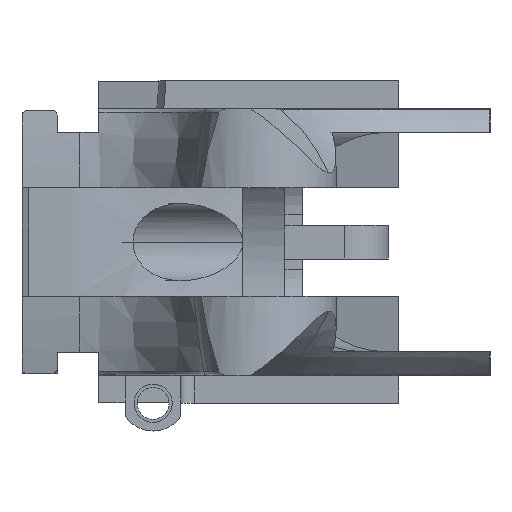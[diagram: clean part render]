
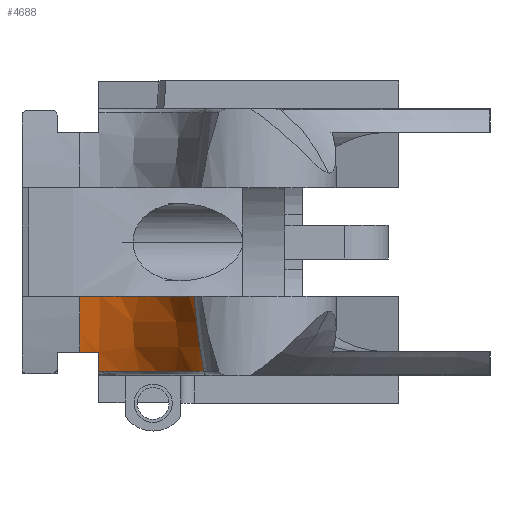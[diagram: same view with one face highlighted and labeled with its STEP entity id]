
A CAD part, left-side view. The second image highlights one B-rep face of the part: STEP entity #4688.
In plain terms, the highlighted free-form (B-spline) face has degree [3, 3] with [4, 4] control points.
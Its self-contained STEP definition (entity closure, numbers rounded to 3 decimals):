
#46 = CARTESIAN_POINT ( 'NONE',  ( -88.521, -1.184, -5.759 ) ) ;
#172 = EDGE_CURVE ( 'NONE', #8084, #7736, #11027, .T. ) ;
#174 = CARTESIAN_POINT ( 'NONE',  ( -77.615, -50.503, 0. ) ) ;
#343 = CARTESIAN_POINT ( 'NONE',  ( -80.423, 5.867, -9.367 ) ) ;
#382 = CARTESIAN_POINT ( 'NONE',  ( -85.981, -1.056, -9.367 ) ) ;
#948 = CARTESIAN_POINT ( 'NONE',  ( -80.848, 2.659, -7.57 ) ) ;
#1007 = CIRCLE ( 'NONE', #6863, 9.392 ) ;
#1082 = DIRECTION ( 'NONE',  ( 0., 0., 1. ) ) ;
#1248 = CARTESIAN_POINT ( 'NONE',  ( -30.319, 7.237, 0. ) ) ;
#1277 = CARTESIAN_POINT ( 'NONE',  ( -87.367, -1.543, -9.367 ) ) ;
#1711 = CARTESIAN_POINT ( 'NONE',  ( -88.325, -1.736, -9.367 ) ) ;
#1758 = CARTESIAN_POINT ( 'NONE',  ( -88.325, -1.736, -9.367 ) ) ;
#1840 = CARTESIAN_POINT ( 'NONE',  ( -88.472, -1.419, -7.57 ) ) ;
#1937 = EDGE_CURVE ( 'NONE', #3901, #10602, #9579, .T. ) ;
#1997 = EDGE_CURVE ( 'NONE', #3901, #7877, #7522, .T. ) ;
#2120 = ORIENTED_EDGE ( 'NONE', *, *, #172, .T. ) ;
#2134 = CARTESIAN_POINT ( 'NONE',  ( -80.652, 4.92, -9.367 ) ) ;
#2142 = DIRECTION ( 'NONE',  ( 0., 0., 1. ) ) ;
#2167 = CARTESIAN_POINT ( 'NONE',  ( -88.325, -1.736, -9.367 ) ) ;
#2214 = AXIS2_PLACEMENT_3D ( 'NONE', #7499, #2228, #8372 ) ;
#2228 = DIRECTION ( 'NONE',  ( 0., 0., 1. ) ) ;
#2232 = CARTESIAN_POINT ( 'NONE',  ( -88.325, -1.736, -9.367 ) ) ;
#2313 = EDGE_CURVE ( 'NONE', #7877, #11165, #3927, .T. ) ;
#2441 = EDGE_CURVE ( 'NONE', #8084, #11165, #6672, .T. ) ;
#2540 = EDGE_CURVE ( 'NONE', #7736, #2739, #8155, .T. ) ;
#2553 = ORIENTED_EDGE ( 'NONE', *, *, #1937, .F. ) ;
#2558 = CARTESIAN_POINT ( 'NONE',  ( -88.479, -1.035, -3.937 ) ) ;
#2729 = CARTESIAN_POINT ( 'NONE',  ( -80.511, 2.493, -9.367 ) ) ;
#2739 = VERTEX_POINT ( 'NONE', #9456 ) ;
#2751 = EDGE_CURVE ( 'NONE', #10602, #2739, #1007, .T. ) ;
#3018 = CARTESIAN_POINT ( 'NONE',  ( -80.994, 4.011, -9.367 ) ) ;
#3075 = CARTESIAN_POINT ( 'NONE',  ( -80.423, 5.867, -9.367 ) ) ;
#3589 = CARTESIAN_POINT ( 'NONE',  ( -84.2, -0.397, -3.937 ) ) ;
#3627 = CARTESIAN_POINT ( 'NONE',  ( -88.402, -1.748, -9.367 ) ) ;
#3901 = VERTEX_POINT ( 'NONE', #5484 ) ;
#3913 = CARTESIAN_POINT ( 'NONE',  ( -81.305, 3.348, -9.367 ) ) ;
#3927 = B_SPLINE_CURVE_WITH_KNOTS ( 'NONE', 3,
 ( #1711, #5273, #7034, #1758 ),
 .UNSPECIFIED., .F., .F.,
 ( 4, 4 ),
 ( 0., 0. ),
 .UNSPECIFIED. ) ;
#4460 = CARTESIAN_POINT ( 'NONE',  ( -80.824, 7.237, -5.759 ) ) ;
#4688 = ADVANCED_FACE ( 'NONE', ( #5041 ), #5638, .T. ) ;
#4791 = CARTESIAN_POINT ( 'NONE',  ( -82.477, 1.514, -9.367 ) ) ;
#4824 = EDGE_LOOP ( 'NONE', ( #2553, #7483, #10392, #8589, #2120, #7102, #5595 ) ) ;
#4846 = CARTESIAN_POINT ( 'NONE',  ( -80.669, 5.867, -7.976 ) ) ;
#5041 = FACE_OUTER_BOUND ( 'NONE', #4824, .T. ) ;
#5125 = CARTESIAN_POINT ( 'NONE',  ( -89.865, 7.772, -7.976 ) ) ;
#5273 = CARTESIAN_POINT ( 'NONE',  ( -88.325, -1.736, -9.367 ) ) ;
#5318 = AXIS2_PLACEMENT_3D ( 'NONE', #174, #6374, #1082 ) ;
#5368 = CARTESIAN_POINT ( 'NONE',  ( -84.102, -0.521, -5.759 ) ) ;
#5484 = CARTESIAN_POINT ( 'NONE',  ( -80.423, 5.867, -9.367 ) ) ;
#5595 = ORIENTED_EDGE ( 'NONE', *, *, #2751, .F. ) ;
#5638 =( BOUNDED_SURFACE ( )  B_SPLINE_SURFACE ( 3, 3, ( 
 ( #7963, #9682, #3589, #9730 ),
 ( #4460, #10614, #5368, #46 ),
 ( #6250, #948, #7124, #1840 ),
 ( #7998, #2729, #8875, #3627 ) ),
 .UNSPECIFIED., .F., .F., .F. ) 
 B_SPLINE_SURFACE_WITH_KNOTS ( ( 4, 4 ),
 ( 4, 4 ),
 ( 0., 1. ),
 ( 0., 1. ),
 .UNSPECIFIED. ) 
 GEOMETRIC_REPRESENTATION_ITEM ( )  RATIONAL_B_SPLINE_SURFACE ( (
 ( 1., 0.851, 0.851, 1.),
 ( 0.999, 0.85, 0.85, 0.999),
 ( 0.999, 0.85, 0.85, 0.999),
 ( 1., 0.851, 0.851, 1.) ) ) 
 REPRESENTATION_ITEM ( '' )  SURFACE ( )  );
#5662 = CARTESIAN_POINT ( 'NONE',  ( -80.52, 5.388, -9.367 ) ) ;
#5700 = CARTESIAN_POINT ( 'NONE',  ( -84.676, -0.401, -9.367 ) ) ;
#6013 = DIRECTION ( 'NONE',  ( -1., 0., 0. ) ) ;
#6250 = CARTESIAN_POINT ( 'NONE',  ( -80.585, 7.237, -7.57 ) ) ;
#6374 = DIRECTION ( 'NONE',  ( -0.977, -0.214, 0. ) ) ;
#6573 = CARTESIAN_POINT ( 'NONE',  ( -86.437, -1.243, -9.367 ) ) ;
#6672 = CIRCLE ( 'NONE', #5318, 50.8 ) ;
#6859 = CARTESIAN_POINT ( 'NONE',  ( -80.669, 5.867, -7.976 ) ) ;
#6863 = AXIS2_PLACEMENT_3D ( 'NONE', #5125, #11261, #6013 ) ;
#7034 = CARTESIAN_POINT ( 'NONE',  ( -88.325, -1.736, -9.367 ) ) ;
#7102 = ORIENTED_EDGE ( 'NONE', *, *, #2540, .T. ) ;
#7124 = CARTESIAN_POINT ( 'NONE',  ( -83.937, -0.731, -7.57 ) ) ;
#7404 = DIRECTION ( 'NONE',  ( 0., -1., 0. ) ) ;
#7434 = CARTESIAN_POINT ( 'NONE',  ( -87.842, -1.658, -9.367 ) ) ;
#7483 = ORIENTED_EDGE ( 'NONE', *, *, #1997, .T. ) ;
#7499 = CARTESIAN_POINT ( 'NONE',  ( -89.865, 7.772, -3.937 ) ) ;
#7522 = B_SPLINE_CURVE_WITH_KNOTS ( 'NONE', 3,
 ( #343, #5662, #2134, #8281, #3018, #9157, #3913, #10038, #4791, #10939, #5700, #382, #6573, #1277, #7434, #2167 ),
 .UNSPECIFIED., .F., .F.,
 ( 4, 2, 2, 2, 2, 2, 2, 4 ),
 ( 0., 0.001, 0.002, 0.003, 0.006, 0.009, 0.01, 0.012 ),
 .UNSPECIFIED. ) ;
#7736 = VERTEX_POINT ( 'NONE', #8200 ) ;
#7877 = VERTEX_POINT ( 'NONE', #2232 ) ;
#7963 = CARTESIAN_POINT ( 'NONE',  ( -80.966, 7.237, -3.937 ) ) ;
#7998 = CARTESIAN_POINT ( 'NONE',  ( -80.248, 7.237, -9.367 ) ) ;
#8084 = VERTEX_POINT ( 'NONE', #2558 ) ;
#8155 = CIRCLE ( 'NONE', #10605, 50.8 ) ;
#8200 = CARTESIAN_POINT ( 'NONE',  ( -80.966, 7.237, -3.937 ) ) ;
#8281 = CARTESIAN_POINT ( 'NONE',  ( -80.902, 4.236, -9.367 ) ) ;
#8336 = CARTESIAN_POINT ( 'NONE',  ( -80.511, 5.867, -8.904 ) ) ;
#8372 = DIRECTION ( 'NONE',  ( -1., 0., 0. ) ) ;
#8589 = ORIENTED_EDGE ( 'NONE', *, *, #2441, .F. ) ;
#8667 = CARTESIAN_POINT ( 'NONE',  ( -88.325, -1.736, -9.367 ) ) ;
#8875 = CARTESIAN_POINT ( 'NONE',  ( -83.705, -1.026, -9.367 ) ) ;
#9157 = CARTESIAN_POINT ( 'NONE',  ( -81.195, 3.568, -9.367 ) ) ;
#9456 = CARTESIAN_POINT ( 'NONE',  ( -80.489, 7.237, -7.976 ) ) ;
#9579 = B_SPLINE_CURVE_WITH_KNOTS ( 'NONE', 3,
 ( #3075, #8336, #10091, #4846 ),
 .UNSPECIFIED., .F., .F.,
 ( 4, 4 ),
 ( 0., 0.002 ),
 .UNSPECIFIED. ) ;
#9682 = CARTESIAN_POINT ( 'NONE',  ( -81.23, 2.847, -3.937 ) ) ;
#9730 = CARTESIAN_POINT ( 'NONE',  ( -88.55, -1.046, -3.937 ) ) ;
#10038 = CARTESIAN_POINT ( 'NONE',  ( -81.891, 2.282, -9.367 ) ) ;
#10091 = CARTESIAN_POINT ( 'NONE',  ( -80.593, 5.867, -8.44 ) ) ;
#10392 = ORIENTED_EDGE ( 'NONE', *, *, #2313, .T. ) ;
#10602 = VERTEX_POINT ( 'NONE', #6859 ) ;
#10605 = AXIS2_PLACEMENT_3D ( 'NONE', #1248, #7404, #2142 ) ;
#10614 = CARTESIAN_POINT ( 'NONE',  ( -81.088, 2.777, -5.759 ) ) ;
#10939 = CARTESIAN_POINT ( 'NONE',  ( -83.887, 0.156, -9.367 ) ) ;
#11027 = CIRCLE ( 'NONE', #2214, 8.916 ) ;
#11165 = VERTEX_POINT ( 'NONE', #8667 ) ;
#11261 = DIRECTION ( 'NONE',  ( 0., 0., 1. ) ) ;
